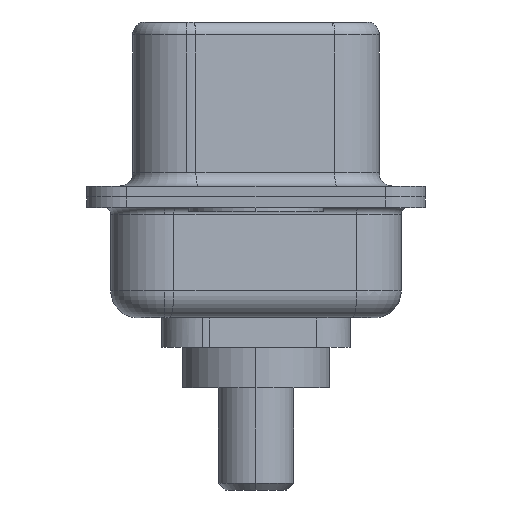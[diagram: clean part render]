
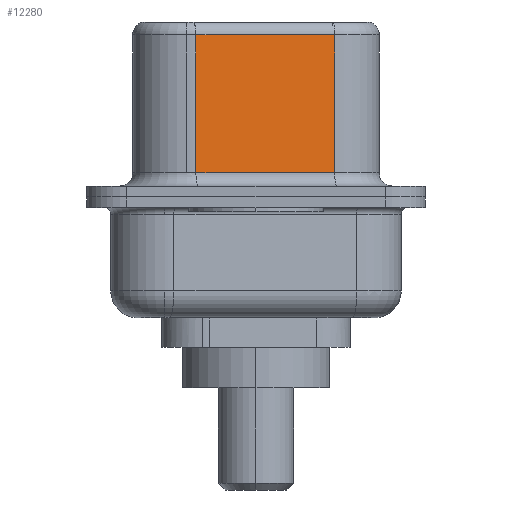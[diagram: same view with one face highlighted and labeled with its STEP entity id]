
A CAD part, left-side view. The second image highlights one B-rep face of the part: STEP entity #12280.
In plain terms, the highlighted planar face has unit normal (-0.985, -0.174, 0).
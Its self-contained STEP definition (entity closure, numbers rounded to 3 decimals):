
#515 = LINE ( 'NONE', #8571, #6320 ) ;
#2953 = DIRECTION ( 'NONE',  ( 0.174, -0.985, 0. ) ) ;
#3440 = ORIENTED_EDGE ( 'NONE', *, *, #7905, .T. ) ;
#3454 = DIRECTION ( 'NONE',  ( 0., 0., -1. ) ) ;
#4008 = VERTEX_POINT ( 'NONE', #8350 ) ;
#4186 = EDGE_CURVE ( 'NONE', #4008, #8465, #11393, .T. ) ;
#4358 = VERTEX_POINT ( 'NONE', #4456 ) ;
#4456 = CARTESIAN_POINT ( 'NONE',  ( 4.58, -2.927, 6.02 ) ) ;
#4469 = EDGE_LOOP ( 'NONE', ( #5297, #3440, #14024, #5191 ) ) ;
#4491 = VECTOR ( 'NONE', #3454, 1000. ) ;
#4704 = EDGE_CURVE ( 'NONE', #4358, #8465, #8082, .T. ) ;
#5191 = ORIENTED_EDGE ( 'NONE', *, *, #4186, .T. ) ;
#5297 = ORIENTED_EDGE ( 'NONE', *, *, #4704, .F. ) ;
#6110 = PLANE ( 'NONE',  #13187 ) ;
#6320 = VECTOR ( 'NONE', #8479, 1000. ) ;
#6345 = VERTEX_POINT ( 'NONE', #9866 ) ;
#6799 = EDGE_CURVE ( 'NONE', #6345, #4008, #8600, .T. ) ;
#7215 = VECTOR ( 'NONE', #8750, 1000. ) ;
#7295 = DIRECTION ( 'NONE',  ( -0.174, 0.985, 0. ) ) ;
#7861 = CARTESIAN_POINT ( 'NONE',  ( 3.67, 2.233, 6.52 ) ) ;
#7905 = EDGE_CURVE ( 'NONE', #4358, #6345, #515, .T. ) ;
#8074 = FACE_OUTER_BOUND ( 'NONE', #4469, .T. ) ;
#8082 = LINE ( 'NONE', #9940, #7215 ) ;
#8271 = CARTESIAN_POINT ( 'NONE',  ( 4.58, -2.927, 6.52 ) ) ;
#8350 = CARTESIAN_POINT ( 'NONE',  ( 3.67, 2.233, 0.9 ) ) ;
#8465 = VERTEX_POINT ( 'NONE', #8498 ) ;
#8479 = DIRECTION ( 'NONE',  ( -0.174, 0.985, 0. ) ) ;
#8498 = CARTESIAN_POINT ( 'NONE',  ( 4.58, -2.927, 0.9 ) ) ;
#8571 = CARTESIAN_POINT ( 'NONE',  ( 4.58, -2.927, 6.02 ) ) ;
#8600 = LINE ( 'NONE', #7861, #4491 ) ;
#8750 = DIRECTION ( 'NONE',  ( 0., 0., -1. ) ) ;
#9170 = CARTESIAN_POINT ( 'NONE',  ( 4.58, -2.927, 0.9 ) ) ;
#9866 = CARTESIAN_POINT ( 'NONE',  ( 3.67, 2.233, 6.02 ) ) ;
#9940 = CARTESIAN_POINT ( 'NONE',  ( 4.58, -2.927, 6.52 ) ) ;
#10481 = DIRECTION ( 'NONE',  ( 0.985, 0.174, 0. ) ) ;
#11032 = VECTOR ( 'NONE', #2953, 1000. ) ;
#11393 = LINE ( 'NONE', #9170, #11032 ) ;
#12280 = ADVANCED_FACE ( 'NONE', ( #8074 ), #6110, .F. ) ;
#13187 = AXIS2_PLACEMENT_3D ( 'NONE', #8271, #10481, #7295 ) ;
#14024 = ORIENTED_EDGE ( 'NONE', *, *, #6799, .T. ) ;
